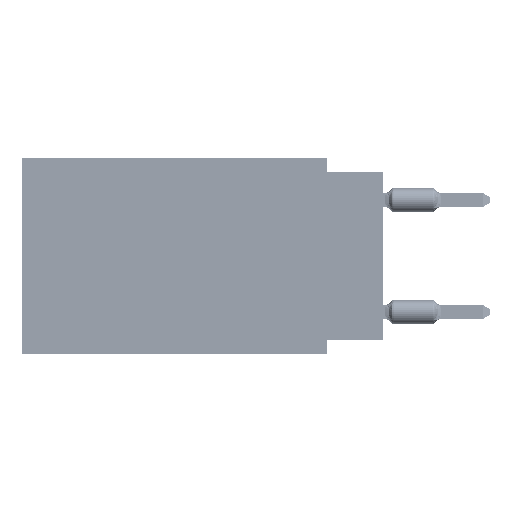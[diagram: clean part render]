
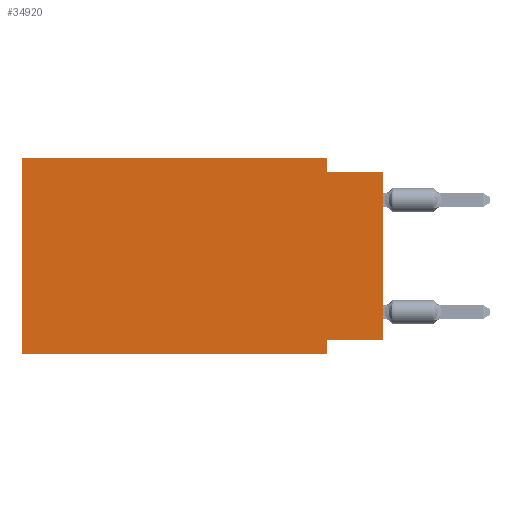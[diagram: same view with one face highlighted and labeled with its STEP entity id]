
A CAD part, left-side view. The second image highlights one B-rep face of the part: STEP entity #34920.
In plain terms, the highlighted planar face has unit normal (-1, 0, 0).
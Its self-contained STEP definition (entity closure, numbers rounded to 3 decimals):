
#1469 = VECTOR ( 'NONE', #4713, 1000. ) ;
#4713 = DIRECTION ( 'NONE',  ( 0., 0., -1. ) ) ;
#4773 = DIRECTION ( 'NONE',  ( 0., 0., -1. ) ) ;
#5135 = CARTESIAN_POINT ( 'NONE',  ( 0., 16.383, 0. ) ) ;
#8923 = EDGE_CURVE ( 'NONE', #25176, #89888, #24643, .T. ) ;
#9542 = CARTESIAN_POINT ( 'NONE',  ( 0., 16.383, 0. ) ) ;
#10738 = CARTESIAN_POINT ( 'NONE',  ( 0., 0., 0. ) ) ;
#13541 = VECTOR ( 'NONE', #67049, 1000. ) ;
#16107 = VECTOR ( 'NONE', #79556, 1000. ) ;
#17017 = ORIENTED_EDGE ( 'NONE', *, *, #27854, .T. ) ;
#17861 = EDGE_CURVE ( 'NONE', #106927, #18885, #87315, .T. ) ;
#18120 = CARTESIAN_POINT ( 'NONE',  ( 0., 16.383, -8.89 ) ) ;
#18244 = CARTESIAN_POINT ( 'NONE',  ( 0., 2.54, -8.89 ) ) ;
#18247 = ORIENTED_EDGE ( 'NONE', *, *, #17861, .F. ) ;
#18615 = EDGE_CURVE ( 'NONE', #33424, #87804, #48772, .T. ) ;
#18885 = VERTEX_POINT ( 'NONE', #80486 ) ;
#21546 = DIRECTION ( 'NONE',  ( 0., 0., -1. ) ) ;
#24022 = EDGE_CURVE ( 'NONE', #25176, #87804, #100220, .T. ) ;
#24643 = LINE ( 'NONE', #5135, #13541 ) ;
#25176 = VERTEX_POINT ( 'NONE', #18120 ) ;
#27854 = EDGE_CURVE ( 'NONE', #57123, #18885, #45490, .T. ) ;
#33424 = VERTEX_POINT ( 'NONE', #68496 ) ;
#34084 = CARTESIAN_POINT ( 'NONE',  ( 0., 0., -0.635 ) ) ;
#34920 = ADVANCED_FACE ( 'NONE', ( #67246 ), #93862, .F. ) ;
#37333 = ORIENTED_EDGE ( 'NONE', *, *, #8923, .F. ) ;
#37759 = CARTESIAN_POINT ( 'NONE',  ( 0., 16.383, -8.89 ) ) ;
#40340 = VECTOR ( 'NONE', #108684, 1000. ) ;
#45490 = LINE ( 'NONE', #10738, #103373 ) ;
#48772 = LINE ( 'NONE', #84040, #54353 ) ;
#49809 = EDGE_CURVE ( 'NONE', #66566, #106927, #102486, .T. ) ;
#51681 = ORIENTED_EDGE ( 'NONE', *, *, #89307, .F. ) ;
#52263 = CARTESIAN_POINT ( 'NONE',  ( 0., 16.383, 0. ) ) ;
#52611 = DIRECTION ( 'NONE',  ( 0., -1., 0. ) ) ;
#54278 = ORIENTED_EDGE ( 'NONE', *, *, #24022, .T. ) ;
#54353 = VECTOR ( 'NONE', #4773, 1000. ) ;
#56287 = CARTESIAN_POINT ( 'NONE',  ( 0., 16.383, 0. ) ) ;
#57123 = VERTEX_POINT ( 'NONE', #75855 ) ;
#57899 = VECTOR ( 'NONE', #52611, 1000. ) ;
#57999 = DIRECTION ( 'NONE',  ( 1., 0., 0. ) ) ;
#65738 = ORIENTED_EDGE ( 'NONE', *, *, #49809, .F. ) ;
#66566 = VERTEX_POINT ( 'NONE', #97503 ) ;
#67049 = DIRECTION ( 'NONE',  ( 0., 0., 1. ) ) ;
#67246 = FACE_OUTER_BOUND ( 'NONE', #76960, .T. ) ;
#68496 = CARTESIAN_POINT ( 'NONE',  ( 0., 2.54, -8.255 ) ) ;
#70594 = ORIENTED_EDGE ( 'NONE', *, *, #96279, .F. ) ;
#74053 = CARTESIAN_POINT ( 'NONE',  ( 0., 2.54, -0.635 ) ) ;
#75855 = CARTESIAN_POINT ( 'NONE',  ( 0., 0., -8.255 ) ) ;
#76960 = EDGE_LOOP ( 'NONE', ( #17017, #18247, #65738, #70594, #37333, #54278, #84384, #51681 ) ) ;
#79556 = DIRECTION ( 'NONE',  ( 0., -1., 0. ) ) ;
#80297 = AXIS2_PLACEMENT_3D ( 'NONE', #56287, #57999, #21546 ) ;
#80486 = CARTESIAN_POINT ( 'NONE',  ( 0., 0., -0.635 ) ) ;
#84040 = CARTESIAN_POINT ( 'NONE',  ( 0., 2.54, -8.89 ) ) ;
#84384 = ORIENTED_EDGE ( 'NONE', *, *, #18615, .F. ) ;
#84609 = DIRECTION ( 'NONE',  ( 0., 0., 1. ) ) ;
#85133 = CARTESIAN_POINT ( 'NONE',  ( 0., 2.54, 0. ) ) ;
#87315 = LINE ( 'NONE', #34084, #57899 ) ;
#87804 = VERTEX_POINT ( 'NONE', #18244 ) ;
#89307 = EDGE_CURVE ( 'NONE', #57123, #33424, #90792, .T. ) ;
#89888 = VERTEX_POINT ( 'NONE', #52263 ) ;
#90792 = LINE ( 'NONE', #100591, #40340 ) ;
#93862 = PLANE ( 'NONE',  #80297 ) ;
#95786 = LINE ( 'NONE', #9542, #16107 ) ;
#96279 = EDGE_CURVE ( 'NONE', #89888, #66566, #95786, .T. ) ;
#97503 = CARTESIAN_POINT ( 'NONE',  ( 0., 2.54, 0. ) ) ;
#99775 = VECTOR ( 'NONE', #107740, 1000. ) ;
#100220 = LINE ( 'NONE', #37759, #99775 ) ;
#100591 = CARTESIAN_POINT ( 'NONE',  ( 0., 0., -8.255 ) ) ;
#102486 = LINE ( 'NONE', #85133, #1469 ) ;
#103373 = VECTOR ( 'NONE', #84609, 1000. ) ;
#106927 = VERTEX_POINT ( 'NONE', #74053 ) ;
#107740 = DIRECTION ( 'NONE',  ( 0., -1., 0. ) ) ;
#108684 = DIRECTION ( 'NONE',  ( 0., 1., 0. ) ) ;
